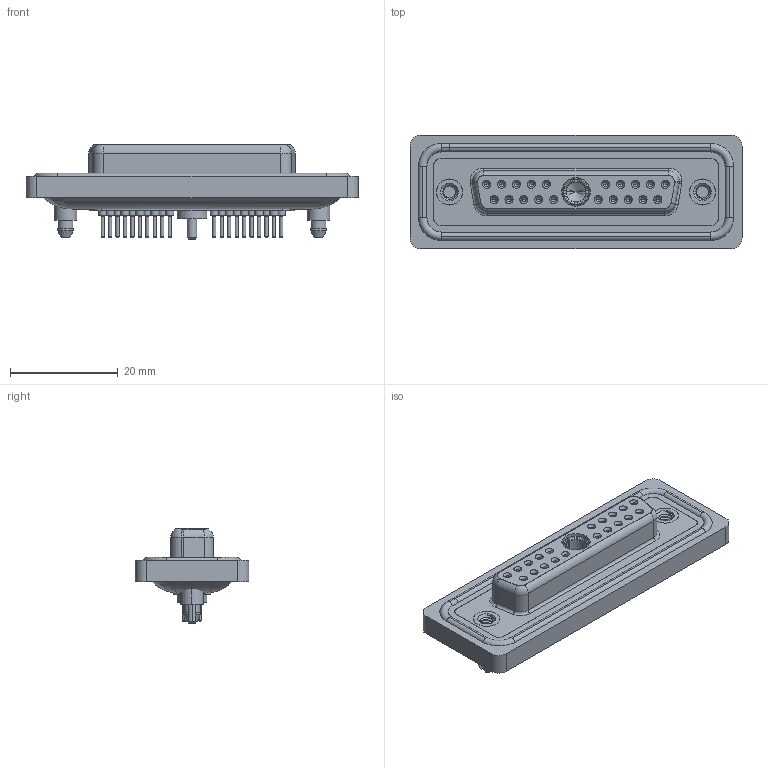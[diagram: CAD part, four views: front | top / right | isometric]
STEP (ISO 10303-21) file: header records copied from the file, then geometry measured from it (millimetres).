
FILE_DESCRIPTION (( 'STEP AP203' ), '1' );
FILE_NAME ('628W21W1324-1N5.STEP', '2024-04-09T22:12:35', ( '' ), ( '' ), 'SwSTEP 2.0', 'SolidWorks 2023', '' );
FILE_SCHEMA (( 'CONFIG_CONTROL_DESIGN' ));
Length unit declared in the file: millimetre
Products named in the file (9): 628Combo Threaded Boardlock_5; 628Combo Housing_21W1; Power Socket_10A S; 628Combo Contact Row 1_24; 628Combo Shell Front_25 Contacts; 628Combo Contact Row 2_24; 628Combo Shell Rear_25 Contacts; 628Combo Waterproof Housing_25 Contacts; 628W21W1324-1N5
Assembly tree (27 placements, depth 2):
  628W21W1324-1N5
    628Combo Housing_21W1
    628Combo Waterproof Housing_25 Contacts
    628Combo Shell Front_25 Contacts
    628Combo Shell Rear_25 Contacts
    628Combo Threaded Boardlock_5  x2
    628Combo Contact Row 1_24  x10
    628Combo Contact Row 2_24  x10
    Power Socket_10A S
Bounding box: 61.75 x 21.1 x 17.55 mm (x, y, z)
Volume: 8493.1 mm3; surface area: 14322.3 mm2
Topology: 29 solids, 29 shells, 1610 faces, 3813 edges, 2359 vertices
Faces by surface type: cylinder 623, plane 450, torus 355, cone 171, bspline 11
Entity records: 26961 total; most frequent: CARTESIAN_POINT 6424, DIRECTION 4321, ORIENTED_EDGE 3776, EDGE_CURVE 1888, AXIS2_PLACEMENT_3D 1789, VERTEX_POINT 1202, CIRCLE 971, EDGE_LOOP 942
